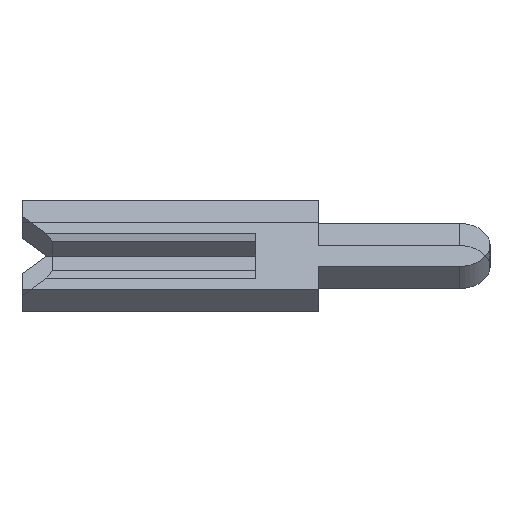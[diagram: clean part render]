
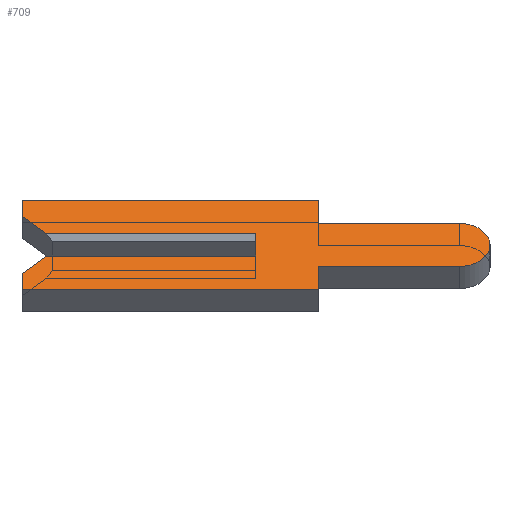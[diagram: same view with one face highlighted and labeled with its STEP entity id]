
A CAD part, left-side view. The second image highlights one B-rep face of the part: STEP entity #709.
In plain terms, the highlighted face is planar.
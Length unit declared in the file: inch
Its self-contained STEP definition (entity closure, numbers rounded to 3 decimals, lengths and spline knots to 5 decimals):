
#52 = VERTEX_POINT ( 'NONE', #774 ) ;
#58 = ORIENTED_EDGE ( 'NONE', *, *, #520, .F. ) ;
#122 = CARTESIAN_POINT ( 'NONE',  ( -0.01, -0.04, 0.04 ) ) ;
#123 = ORIENTED_EDGE ( 'NONE', *, *, #413, .F. ) ;
#129 = AXIS2_PLACEMENT_3D ( 'NONE', #1600, #880, #340 ) ;
#149 = VERTEX_POINT ( 'NONE', #2942 ) ;
#213 = ORIENTED_EDGE ( 'NONE', *, *, #2652, .F. ) ;
#221 = VERTEX_POINT ( 'NONE', #601 ) ;
#242 = CARTESIAN_POINT ( 'NONE',  ( -0.01, 0.15, 0.04 ) ) ;
#253 = VECTOR ( 'NONE', #3145, 39.37008 ) ;
#254 = DIRECTION ( 'NONE',  ( 0., 1., 0. ) ) ;
#281 = DIRECTION ( 'NONE',  ( 0., 0., 1. ) ) ;
#311 = VERTEX_POINT ( 'NONE', #2413 ) ;
#340 = DIRECTION ( 'NONE',  ( 0., 0., -1. ) ) ;
#354 = LINE ( 'NONE', #242, #972 ) ;
#368 = LINE ( 'NONE', #1991, #1652 ) ;
#413 = EDGE_CURVE ( 'NONE', #2922, #2245, #2114, .T. ) ;
#418 = CARTESIAN_POINT ( 'NONE',  ( -0.01, -0.04, -0.04 ) ) ;
#449 = VECTOR ( 'NONE', #1363, 39.37008 ) ;
#520 = EDGE_CURVE ( 'NONE', #3346, #311, #1052, .T. ) ;
#521 = CARTESIAN_POINT ( 'NONE',  ( -0.01, -0.1305, -0.01 ) ) ;
#545 = CARTESIAN_POINT ( 'NONE',  ( -0.01, 0.1305, 0.0065 ) ) ;
#585 = VERTEX_POINT ( 'NONE', #2278 ) ;
#601 = CARTESIAN_POINT ( 'NONE',  ( -0.01, 0.15, -0.04 ) ) ;
#641 = VERTEX_POINT ( 'NONE', #122 ) ;
#662 = DIRECTION ( 'NONE',  ( 0., 0., -1. ) ) ;
#709 = ADVANCED_FACE ( 'NONE', ( #1081 ), #2811, .F. ) ;
#716 = CARTESIAN_POINT ( 'NONE',  ( -0.01, 0., 0.0065 ) ) ;
#756 = CARTESIAN_POINT ( 'NONE',  ( -0.01, -0.1305, -0.0195 ) ) ;
#769 = CARTESIAN_POINT ( 'NONE',  ( -0.01, 0.15, 0.026 ) ) ;
#774 = CARTESIAN_POINT ( 'NONE',  ( -0.01, 0.15, 0.04 ) ) ;
#794 = DIRECTION ( 'NONE',  ( 0., 0., 1. ) ) ;
#804 = DIRECTION ( 'NONE',  ( 0., 0.707, 0.707 ) ) ;
#812 = VERTEX_POINT ( 'NONE', #418 ) ;
#819 = CARTESIAN_POINT ( 'NONE',  ( -0.01, 0.15, -0.026 ) ) ;
#849 = ORIENTED_EDGE ( 'NONE', *, *, #2732, .F. ) ;
#880 = DIRECTION ( 'NONE',  ( 1., 0., 0. ) ) ;
#892 = LINE ( 'NONE', #1526, #2962 ) ;
#896 = VERTEX_POINT ( 'NONE', #1196 ) ;
#923 = AXIS2_PLACEMENT_3D ( 'NONE', #2011, #951, #662 ) ;
#925 = CARTESIAN_POINT ( 'NONE',  ( -0.01, -0.04, 0.0195 ) ) ;
#940 = VERTEX_POINT ( 'NONE', #925 ) ;
#951 = DIRECTION ( 'NONE',  ( 1., 0., 0. ) ) ;
#972 = VECTOR ( 'NONE', #2143, 39.37008 ) ;
#1014 = DIRECTION ( 'NONE',  ( 0., 1., 0. ) ) ;
#1020 = DIRECTION ( 'NONE',  ( 0., 0., -1. ) ) ;
#1052 = LINE ( 'NONE', #716, #253 ) ;
#1080 = DIRECTION ( 'NONE',  ( 0., 0., -1. ) ) ;
#1081 = FACE_OUTER_BOUND ( 'NONE', #3099, .T. ) ;
#1132 = EDGE_CURVE ( 'NONE', #149, #812, #1332, .T. ) ;
#1192 = ORIENTED_EDGE ( 'NONE', *, *, #2220, .F. ) ;
#1196 = CARTESIAN_POINT ( 'NONE',  ( -0.01, 0.134, 0.01 ) ) ;
#1210 = EDGE_CURVE ( 'NONE', #585, #2871, #2144, .T. ) ;
#1332 = LINE ( 'NONE', #1350, #2599 ) ;
#1350 = CARTESIAN_POINT ( 'NONE',  ( -0.01, -0.04, -0.04 ) ) ;
#1358 = ORIENTED_EDGE ( 'NONE', *, *, #2833, .F. ) ;
#1362 = VERTEX_POINT ( 'NONE', #2966 ) ;
#1363 = DIRECTION ( 'NONE',  ( 0., -0.707, 0.707 ) ) ;
#1415 = ORIENTED_EDGE ( 'NONE', *, *, #1653, .F. ) ;
#1480 = ORIENTED_EDGE ( 'NONE', *, *, #2577, .F. ) ;
#1526 = CARTESIAN_POINT ( 'NONE',  ( -0.01, 0.15, -0.04 ) ) ;
#1600 = CARTESIAN_POINT ( 'NONE',  ( -0.01, -0.1305, 0. ) ) ;
#1615 = LINE ( 'NONE', #1803, #2330 ) ;
#1618 = VECTOR ( 'NONE', #281, 39.37008 ) ;
#1652 = VECTOR ( 'NONE', #1014, 39.37008 ) ;
#1653 = EDGE_CURVE ( 'NONE', #2245, #149, #368, .T. ) ;
#1803 = CARTESIAN_POINT ( 'NONE',  ( -0.01, -0.04, 0.04 ) ) ;
#1820 = VECTOR ( 'NONE', #804, 39.37008 ) ;
#1841 = DIRECTION ( 'NONE',  ( 0., -1., 0. ) ) ;
#1905 = CARTESIAN_POINT ( 'NONE',  ( -0.01, 0.15, 0.01 ) ) ;
#1908 = CARTESIAN_POINT ( 'NONE',  ( -0.01, 0.1305, -0.0065 ) ) ;
#1991 = CARTESIAN_POINT ( 'NONE',  ( -0.01, -0.04, -0.0195 ) ) ;
#2011 = CARTESIAN_POINT ( 'NONE',  ( -0.01, -0.1305, 0. ) ) ;
#2046 = VECTOR ( 'NONE', #1841, 39.37008 ) ;
#2072 = ORIENTED_EDGE ( 'NONE', *, *, #3269, .T. ) ;
#2112 = CARTESIAN_POINT ( 'NONE',  ( -0.01, 0.134, -0.01 ) ) ;
#2114 = CIRCLE ( 'NONE', #129, 0.0195 ) ;
#2143 = DIRECTION ( 'NONE',  ( 0., -1., 0. ) ) ;
#2144 = LINE ( 'NONE', #1908, #449 ) ;
#2188 = DIRECTION ( 'NONE',  ( 0., -1., 0. ) ) ;
#2197 = EDGE_CURVE ( 'NONE', #641, #940, #1615, .T. ) ;
#2220 = EDGE_CURVE ( 'NONE', #940, #2922, #2586, .T. ) ;
#2245 = VERTEX_POINT ( 'NONE', #756 ) ;
#2249 = LINE ( 'NONE', #1905, #3324 ) ;
#2278 = CARTESIAN_POINT ( 'NONE',  ( -0.01, 0.15, -0.026 ) ) ;
#2330 = VECTOR ( 'NONE', #1020, 39.37008 ) ;
#2334 = LINE ( 'NONE', #819, #3045 ) ;
#2413 = CARTESIAN_POINT ( 'NONE',  ( -0.01, 0., 0.01 ) ) ;
#2440 = CARTESIAN_POINT ( 'NONE',  ( -0.01, -0.1305, 0.0195 ) ) ;
#2478 = ORIENTED_EDGE ( 'NONE', *, *, #3089, .F. ) ;
#2544 = LINE ( 'NONE', #769, #1618 ) ;
#2555 = EDGE_CURVE ( 'NONE', #52, #641, #354, .T. ) ;
#2567 = LINE ( 'NONE', #545, #1820 ) ;
#2577 = EDGE_CURVE ( 'NONE', #812, #221, #892, .T. ) ;
#2586 = LINE ( 'NONE', #2640, #2751 ) ;
#2599 = VECTOR ( 'NONE', #1080, 39.37008 ) ;
#2640 = CARTESIAN_POINT ( 'NONE',  ( -0.01, -0.04, 0.0195 ) ) ;
#2652 = EDGE_CURVE ( 'NONE', #2871, #3346, #3208, .T. ) ;
#2732 = EDGE_CURVE ( 'NONE', #1362, #52, #2544, .T. ) ;
#2751 = VECTOR ( 'NONE', #2897, 39.37008 ) ;
#2811 = PLANE ( 'NONE',  #923 ) ;
#2833 = EDGE_CURVE ( 'NONE', #221, #585, #2334, .T. ) ;
#2841 = ORIENTED_EDGE ( 'NONE', *, *, #1210, .F. ) ;
#2871 = VERTEX_POINT ( 'NONE', #2112 ) ;
#2897 = DIRECTION ( 'NONE',  ( 0., -1., 0. ) ) ;
#2913 = ORIENTED_EDGE ( 'NONE', *, *, #1132, .F. ) ;
#2922 = VERTEX_POINT ( 'NONE', #2440 ) ;
#2942 = CARTESIAN_POINT ( 'NONE',  ( -0.01, -0.04, -0.0195 ) ) ;
#2961 = ORIENTED_EDGE ( 'NONE', *, *, #2555, .F. ) ;
#2962 = VECTOR ( 'NONE', #254, 39.37008 ) ;
#2966 = CARTESIAN_POINT ( 'NONE',  ( -0.01, 0.15, 0.026 ) ) ;
#3045 = VECTOR ( 'NONE', #794, 39.37008 ) ;
#3089 = EDGE_CURVE ( 'NONE', #896, #1362, #2567, .T. ) ;
#3099 = EDGE_LOOP ( 'NONE', ( #2072, #58, #213, #2841, #1358, #1480, #2913, #1415, #123, #1192, #3154, #2961, #849, #2478 ) ) ;
#3145 = DIRECTION ( 'NONE',  ( 0., 0., 1. ) ) ;
#3154 = ORIENTED_EDGE ( 'NONE', *, *, #2197, .F. ) ;
#3208 = LINE ( 'NONE', #521, #2046 ) ;
#3250 = CARTESIAN_POINT ( 'NONE',  ( -0.01, 0., -0.01 ) ) ;
#3269 = EDGE_CURVE ( 'NONE', #896, #311, #2249, .T. ) ;
#3324 = VECTOR ( 'NONE', #2188, 39.37008 ) ;
#3346 = VERTEX_POINT ( 'NONE', #3250 ) ;
